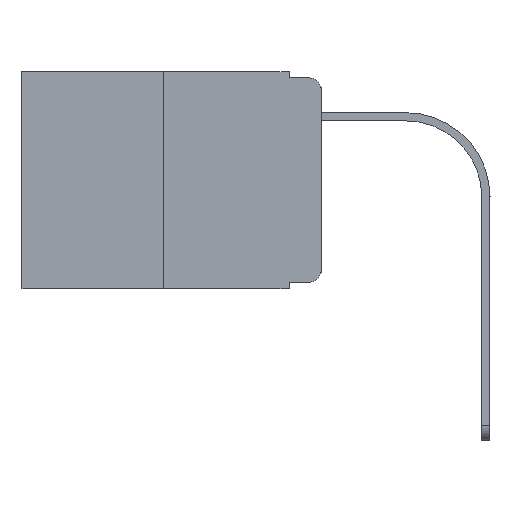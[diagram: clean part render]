
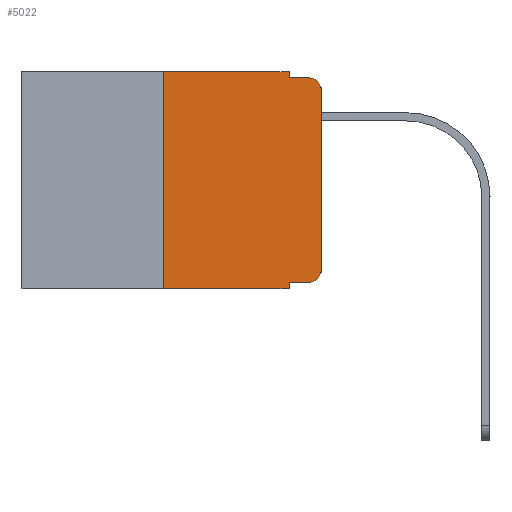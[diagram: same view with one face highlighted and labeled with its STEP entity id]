
A CAD part, left-side view. The second image highlights one B-rep face of the part: STEP entity #5022.
In plain terms, the highlighted planar face has unit normal (-1, 0, 0).
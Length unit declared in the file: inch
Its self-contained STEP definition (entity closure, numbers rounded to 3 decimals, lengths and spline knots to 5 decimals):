
#67 = VECTOR ( 'NONE', #20577, 39.37008 ) ;
#115 = DIRECTION ( 'NONE',  ( 0., -1., 0. ) ) ;
#201 = CARTESIAN_POINT ( 'NONE',  ( 0., 0.25, -0.343 ) ) ;
#769 = DIRECTION ( 'NONE',  ( 0., 0., 1. ) ) ;
#974 = CARTESIAN_POINT ( 'NONE',  ( 0., 0., -0.03 ) ) ;
#1278 = CARTESIAN_POINT ( 'NONE',  ( 0., 0.473, -0.343 ) ) ;
#1574 = EDGE_LOOP ( 'NONE', ( #4769, #17376, #7552, #16714, #4624, #18570, #6741, #6381, #15638, #15459 ) ) ;
#1951 = LINE ( 'NONE', #14704, #17530 ) ;
#2106 = EDGE_CURVE ( 'NONE', #7572, #2419, #10813, .T. ) ;
#2127 = VERTEX_POINT ( 'NONE', #12004 ) ;
#2416 = VERTEX_POINT ( 'NONE', #201 ) ;
#2419 = VERTEX_POINT ( 'NONE', #6725 ) ;
#2593 = VERTEX_POINT ( 'NONE', #4063 ) ;
#3417 = CARTESIAN_POINT ( 'NONE',  ( 0., 0., 0. ) ) ;
#3957 = DIRECTION ( 'NONE',  ( -1., 0., 0. ) ) ;
#4063 = CARTESIAN_POINT ( 'NONE',  ( 0., 0.25, 0. ) ) ;
#4277 = VECTOR ( 'NONE', #4703, 39.37008 ) ;
#4308 = EDGE_CURVE ( 'NONE', #2419, #5232, #11680, .T. ) ;
#4438 = CARTESIAN_POINT ( 'NONE',  ( 0., 0.051, -0.343 ) ) ;
#4624 = ORIENTED_EDGE ( 'NONE', *, *, #19610, .F. ) ;
#4703 = DIRECTION ( 'NONE',  ( 0., -1., 0. ) ) ;
#4769 = ORIENTED_EDGE ( 'NONE', *, *, #8639, .T. ) ;
#4776 = DIRECTION ( 'NONE',  ( 1., 0., 0. ) ) ;
#4835 = VERTEX_POINT ( 'NONE', #14003 ) ;
#5022 = ADVANCED_FACE ( 'NONE', ( #17420 ), #14419, .F. ) ;
#5153 = DIRECTION ( 'NONE',  ( 0., 0., -1. ) ) ;
#5232 = VERTEX_POINT ( 'NONE', #8391 ) ;
#5579 = CARTESIAN_POINT ( 'NONE',  ( 0., 0.25, 0. ) ) ;
#5614 = VERTEX_POINT ( 'NONE', #11475 ) ;
#5641 = EDGE_CURVE ( 'NONE', #4835, #11235, #1951, .T. ) ;
#5786 = CARTESIAN_POINT ( 'NONE',  ( 0., 0.051, 0. ) ) ;
#5897 = VECTOR ( 'NONE', #9933, 39.37008 ) ;
#6381 = ORIENTED_EDGE ( 'NONE', *, *, #5641, .F. ) ;
#6442 = CARTESIAN_POINT ( 'NONE',  ( 0., 0.051, -0.01 ) ) ;
#6725 = CARTESIAN_POINT ( 'NONE',  ( 0., 0.051, -0.01 ) ) ;
#6741 = ORIENTED_EDGE ( 'NONE', *, *, #14734, .T. ) ;
#7552 = ORIENTED_EDGE ( 'NONE', *, *, #4308, .F. ) ;
#7572 = VERTEX_POINT ( 'NONE', #13105 ) ;
#8096 = EDGE_CURVE ( 'NONE', #4835, #2127, #16184, .T. ) ;
#8391 = CARTESIAN_POINT ( 'NONE',  ( 0., 0.02, -0.01 ) ) ;
#8639 = EDGE_CURVE ( 'NONE', #5614, #14192, #15199, .T. ) ;
#9030 = VECTOR ( 'NONE', #11470, 39.37008 ) ;
#9412 = AXIS2_PLACEMENT_3D ( 'NONE', #19224, #4776, #12484 ) ;
#9933 = DIRECTION ( 'NONE',  ( 0., 0., 1. ) ) ;
#10077 = CIRCLE ( 'NONE', #11453, 0.02 ) ;
#10480 = DIRECTION ( 'NONE',  ( 0., 0., -1. ) ) ;
#10813 = LINE ( 'NONE', #5786, #16106 ) ;
#11235 = VERTEX_POINT ( 'NONE', #4438 ) ;
#11453 = AXIS2_PLACEMENT_3D ( 'NONE', #11927, #12138, #13321 ) ;
#11470 = DIRECTION ( 'NONE',  ( 0., -1., 0. ) ) ;
#11475 = CARTESIAN_POINT ( 'NONE',  ( 0., 0., -0.313 ) ) ;
#11533 = LINE ( 'NONE', #1278, #4277 ) ;
#11680 = LINE ( 'NONE', #6442, #14699 ) ;
#11927 = CARTESIAN_POINT ( 'NONE',  ( 0., 0.02, -0.03 ) ) ;
#12004 = CARTESIAN_POINT ( 'NONE',  ( 0., 0.02, -0.333 ) ) ;
#12110 = EDGE_CURVE ( 'NONE', #2127, #5614, #13920, .T. ) ;
#12138 = DIRECTION ( 'NONE',  ( -1., 0., 0. ) ) ;
#12484 = DIRECTION ( 'NONE',  ( 0., 0., -1. ) ) ;
#12805 = CARTESIAN_POINT ( 'NONE',  ( 0., 0.02, -0.313 ) ) ;
#13105 = CARTESIAN_POINT ( 'NONE',  ( 0., 0.051, 0. ) ) ;
#13321 = DIRECTION ( 'NONE',  ( 0., 0., -1. ) ) ;
#13920 = CIRCLE ( 'NONE', #18013, 0.02 ) ;
#14003 = CARTESIAN_POINT ( 'NONE',  ( 0., 0.051, -0.333 ) ) ;
#14070 = CARTESIAN_POINT ( 'NONE',  ( 0., 0.473, 0. ) ) ;
#14192 = VERTEX_POINT ( 'NONE', #974 ) ;
#14419 = PLANE ( 'NONE',  #9412 ) ;
#14699 = VECTOR ( 'NONE', #115, 39.37008 ) ;
#14704 = CARTESIAN_POINT ( 'NONE',  ( 0., 0.051, 0. ) ) ;
#14734 = EDGE_CURVE ( 'NONE', #2416, #11235, #11533, .T. ) ;
#15183 = EDGE_CURVE ( 'NONE', #14192, #5232, #10077, .T. ) ;
#15199 = LINE ( 'NONE', #3417, #5897 ) ;
#15459 = ORIENTED_EDGE ( 'NONE', *, *, #12110, .T. ) ;
#15638 = ORIENTED_EDGE ( 'NONE', *, *, #8096, .T. ) ;
#16106 = VECTOR ( 'NONE', #18853, 39.37008 ) ;
#16184 = LINE ( 'NONE', #19508, #9030 ) ;
#16204 = EDGE_CURVE ( 'NONE', #2416, #2593, #18967, .T. ) ;
#16714 = ORIENTED_EDGE ( 'NONE', *, *, #2106, .F. ) ;
#17167 = LINE ( 'NONE', #14070, #67 ) ;
#17376 = ORIENTED_EDGE ( 'NONE', *, *, #15183, .T. ) ;
#17420 = FACE_OUTER_BOUND ( 'NONE', #1574, .T. ) ;
#17530 = VECTOR ( 'NONE', #5153, 39.37008 ) ;
#18013 = AXIS2_PLACEMENT_3D ( 'NONE', #12805, #3957, #10480 ) ;
#18570 = ORIENTED_EDGE ( 'NONE', *, *, #16204, .F. ) ;
#18674 = VECTOR ( 'NONE', #769, 39.37008 ) ;
#18853 = DIRECTION ( 'NONE',  ( 0., 0., -1. ) ) ;
#18967 = LINE ( 'NONE', #5579, #18674 ) ;
#19224 = CARTESIAN_POINT ( 'NONE',  ( 0., 0.473, 0. ) ) ;
#19508 = CARTESIAN_POINT ( 'NONE',  ( 0., 0.051, -0.333 ) ) ;
#19610 = EDGE_CURVE ( 'NONE', #2593, #7572, #17167, .T. ) ;
#20577 = DIRECTION ( 'NONE',  ( 0., -1., 0. ) ) ;
